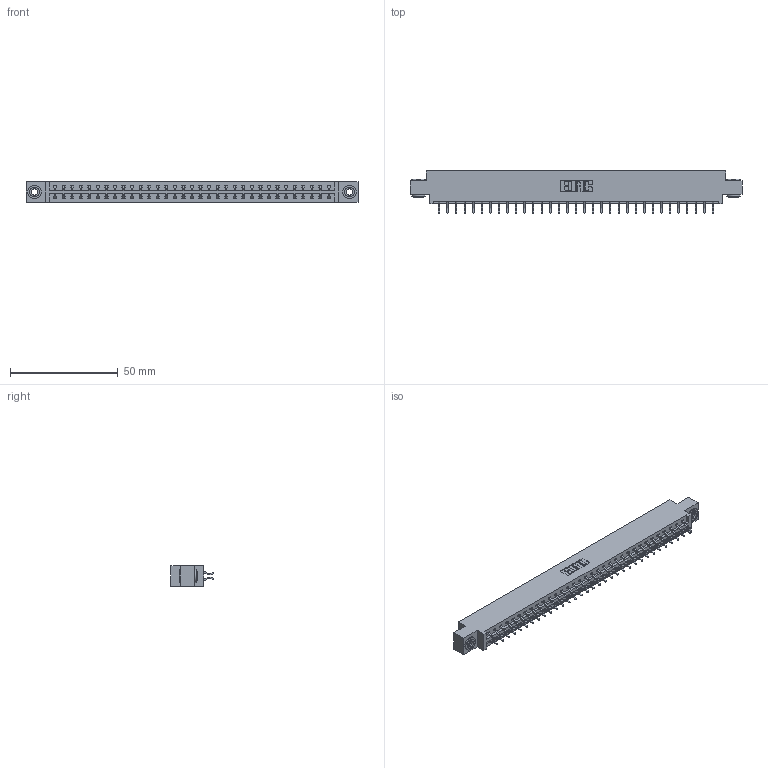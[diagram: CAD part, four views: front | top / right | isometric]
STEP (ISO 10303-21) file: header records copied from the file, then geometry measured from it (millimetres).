
FILE_DESCRIPTION (( 'STEP AP203' ), '1' );
FILE_NAME ('337-066-556-803.STEP', '2019-10-12T01:19:16', ( '' ), ( '' ), 'SwSTEP 2.0', 'SolidWorks 2016', '' );
FILE_SCHEMA (( 'CONFIG_CONTROL_DESIGN' ));
Length unit declared in the file: inch
Products named in the file (4): 337-066-556-803; 345-250-002_345-250-002-102; 337 Part_0.170 Offset - 0.156 Dia-TH; 345-292-001_556 Tail
Assembly tree (69 placements, depth 2):
  337-066-556-803
    337 Part_0.170 Offset - 0.156 Dia-TH
    345-292-001_556 Tail  x66
    345-250-002_345-250-002-102  x2
Bounding box: 153.77 x 19.57 x 9.4 mm (x, y, z)
Volume: 15985.1 mm3; surface area: 18246.4 mm2
Topology: 69 solids, 69 shells, 4116 faces, 12213 edges, 8050 vertices
Faces by surface type: plane 2856, cylinder 1252, cone 8
Entity records: 27752 total; most frequent: CARTESIAN_POINT 4673, ORIENTED_EDGE 4590, DIRECTION 4013, EDGE_CURVE 2295, VECTOR 2135, LINE 2135, VERTEX_POINT 1526, AXIS2_PLACEMENT_3D 939
